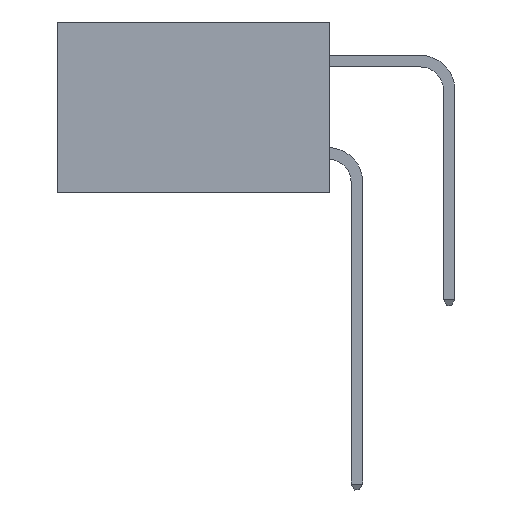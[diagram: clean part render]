
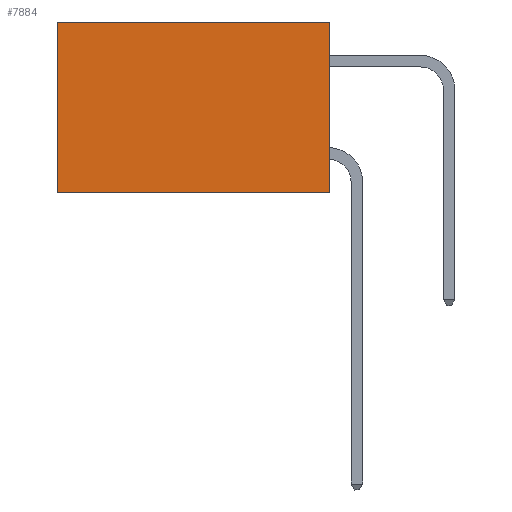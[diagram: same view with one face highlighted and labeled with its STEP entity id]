
A CAD part, left-side view. The second image highlights one B-rep face of the part: STEP entity #7884.
In plain terms, the highlighted planar face has unit normal (-1, 0, 0).
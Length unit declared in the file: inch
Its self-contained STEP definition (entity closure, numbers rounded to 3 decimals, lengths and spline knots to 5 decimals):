
#257 = VERTEX_POINT ( 'NONE', #2212 ) ;
#343 = EDGE_LOOP ( 'NONE', ( #4646, #8691, #812, #4887 ) ) ;
#812 = ORIENTED_EDGE ( 'NONE', *, *, #9659, .F. ) ;
#1294 = VECTOR ( 'NONE', #3756, 39.37008 ) ;
#1765 = VERTEX_POINT ( 'NONE', #5951 ) ;
#1854 = VERTEX_POINT ( 'NONE', #9081 ) ;
#1990 = CARTESIAN_POINT ( 'NONE',  ( 0.277, 0., -0.37 ) ) ;
#2212 = CARTESIAN_POINT ( 'NONE',  ( 0.277, 0.59, -0.37 ) ) ;
#2700 = DIRECTION ( 'NONE',  ( 0., 0., -1. ) ) ;
#2735 = DIRECTION ( 'NONE',  ( 0., 0., -1. ) ) ;
#2893 = EDGE_CURVE ( 'NONE', #1765, #1854, #3336, .T. ) ;
#2970 = VECTOR ( 'NONE', #2700, 39.37008 ) ;
#3336 = LINE ( 'NONE', #4915, #1294 ) ;
#3756 = DIRECTION ( 'NONE',  ( 0., 1., 0. ) ) ;
#3885 = VECTOR ( 'NONE', #5912, 39.37008 ) ;
#4172 = CARTESIAN_POINT ( 'NONE',  ( 0.277, 0., -0.37 ) ) ;
#4200 = PLANE ( 'NONE',  #5118 ) ;
#4465 = EDGE_CURVE ( 'NONE', #5676, #257, #9609, .T. ) ;
#4646 = ORIENTED_EDGE ( 'NONE', *, *, #4721, .T. ) ;
#4721 = EDGE_CURVE ( 'NONE', #1854, #257, #9621, .T. ) ;
#4887 = ORIENTED_EDGE ( 'NONE', *, *, #2893, .T. ) ;
#4915 = CARTESIAN_POINT ( 'NONE',  ( 0.277, 0., 0. ) ) ;
#4978 = LINE ( 'NONE', #4172, #2970 ) ;
#5118 = AXIS2_PLACEMENT_3D ( 'NONE', #1990, #7317, #2735 ) ;
#5676 = VERTEX_POINT ( 'NONE', #5895 ) ;
#5818 = CARTESIAN_POINT ( 'NONE',  ( 0.277, 0.59, -0.37 ) ) ;
#5895 = CARTESIAN_POINT ( 'NONE',  ( 0.277, 0., -0.37 ) ) ;
#5912 = DIRECTION ( 'NONE',  ( 0., 0., -1. ) ) ;
#5951 = CARTESIAN_POINT ( 'NONE',  ( 0.277, 0., 0. ) ) ;
#7317 = DIRECTION ( 'NONE',  ( 1., 0., 0. ) ) ;
#7884 = ADVANCED_FACE ( 'NONE', ( #9778 ), #4200, .F. ) ;
#7984 = VECTOR ( 'NONE', #9239, 39.37008 ) ;
#8691 = ORIENTED_EDGE ( 'NONE', *, *, #4465, .F. ) ;
#9081 = CARTESIAN_POINT ( 'NONE',  ( 0.277, 0.59, 0. ) ) ;
#9239 = DIRECTION ( 'NONE',  ( 0., 1., 0. ) ) ;
#9262 = CARTESIAN_POINT ( 'NONE',  ( 0.277, 0., -0.37 ) ) ;
#9609 = LINE ( 'NONE', #9262, #7984 ) ;
#9621 = LINE ( 'NONE', #5818, #3885 ) ;
#9659 = EDGE_CURVE ( 'NONE', #1765, #5676, #4978, .T. ) ;
#9778 = FACE_OUTER_BOUND ( 'NONE', #343, .T. ) ;
